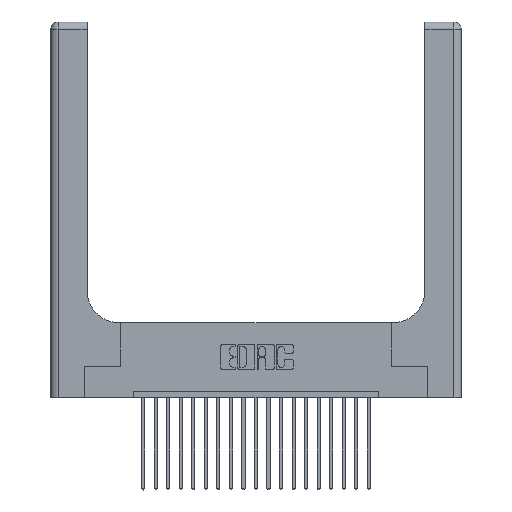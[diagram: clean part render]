
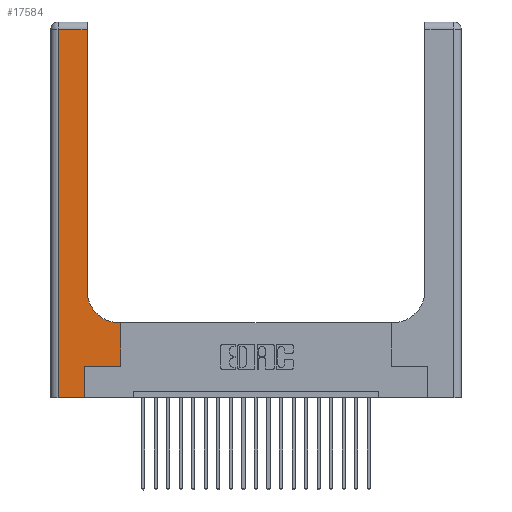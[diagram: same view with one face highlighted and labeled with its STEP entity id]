
A CAD part, top view. The second image highlights one B-rep face of the part: STEP entity #17584.
In plain terms, the highlighted planar face has unit normal (0, 0, 1).
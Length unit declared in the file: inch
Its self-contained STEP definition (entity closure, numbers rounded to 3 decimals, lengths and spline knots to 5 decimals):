
#168 = EDGE_CURVE ( 'NONE', #10191, #3709, #19408, .T. ) ;
#273 = CARTESIAN_POINT ( 'NONE',  ( 0.269, 0.25, 0.37 ) ) ;
#322 = CARTESIAN_POINT ( 'NONE',  ( 0.2915, 3., 0.37 ) ) ;
#757 = DIRECTION ( 'NONE',  ( -1., 0., 0. ) ) ;
#810 = CARTESIAN_POINT ( 'NONE',  ( 0.5585, 0.25, 0.37 ) ) ;
#891 = VERTEX_POINT ( 'NONE', #18353 ) ;
#1217 = VERTEX_POINT ( 'NONE', #17663 ) ;
#1463 = ORIENTED_EDGE ( 'NONE', *, *, #18354, .T. ) ;
#1999 = PLANE ( 'NONE',  #11865 ) ;
#2296 = VERTEX_POINT ( 'NONE', #17834 ) ;
#2933 = CARTESIAN_POINT ( 'NONE',  ( 0.5415, 0.6, 0.37 ) ) ;
#3009 = LINE ( 'NONE', #12864, #11711 ) ;
#3451 = VERTEX_POINT ( 'NONE', #3550 ) ;
#3550 = CARTESIAN_POINT ( 'NONE',  ( 0.5585, 0.25, 0.37 ) ) ;
#3689 = EDGE_CURVE ( 'NONE', #1217, #2296, #17330, .T. ) ;
#3709 = VERTEX_POINT ( 'NONE', #2933 ) ;
#3733 = CARTESIAN_POINT ( 'NONE',  ( 0.5415, 0.85, 0.37 ) ) ;
#3971 = DIRECTION ( 'NONE',  ( 0., 1., 0. ) ) ;
#4291 = DIRECTION ( 'NONE',  ( -1., 0., 0. ) ) ;
#4514 = CARTESIAN_POINT ( 'NONE',  ( 0.269, 0., 0.37 ) ) ;
#4604 = DIRECTION ( 'NONE',  ( 0., -1., 0. ) ) ;
#5093 = EDGE_LOOP ( 'NONE', ( #12547, #1463, #9189, #16789, #19418, #16850, #10582, #7825, #8293 ) ) ;
#5188 = EDGE_CURVE ( 'NONE', #3709, #891, #14259, .T. ) ;
#5521 = DIRECTION ( 'NONE',  ( -1., 0., 0. ) ) ;
#5680 = EDGE_CURVE ( 'NONE', #13908, #3451, #15367, .T. ) ;
#7825 = ORIENTED_EDGE ( 'NONE', *, *, #168, .T. ) ;
#8068 = DIRECTION ( 'NONE',  ( 0., 1., 0. ) ) ;
#8293 = ORIENTED_EDGE ( 'NONE', *, *, #5188, .T. ) ;
#9189 = ORIENTED_EDGE ( 'NONE', *, *, #3689, .T. ) ;
#9375 = EDGE_CURVE ( 'NONE', #891, #15119, #11954, .T. ) ;
#9496 = AXIS2_PLACEMENT_3D ( 'NONE', #3733, #15898, #17657 ) ;
#10011 = DIRECTION ( 'NONE',  ( 1., 0., 0. ) ) ;
#10191 = VERTEX_POINT ( 'NONE', #20766 ) ;
#10582 = ORIENTED_EDGE ( 'NONE', *, *, #22367, .T. ) ;
#10613 = VECTOR ( 'NONE', #10011, 39.37008 ) ;
#11036 = CARTESIAN_POINT ( 'NONE',  ( 0.269, 0., 0.37 ) ) ;
#11158 = LINE ( 'NONE', #20185, #10613 ) ;
#11194 = CARTESIAN_POINT ( 'NONE',  ( 0.269, 0.25, 0.37 ) ) ;
#11668 = VERTEX_POINT ( 'NONE', #4514 ) ;
#11711 = VECTOR ( 'NONE', #757, 39.37008 ) ;
#11865 = AXIS2_PLACEMENT_3D ( 'NONE', #14187, #12590, #5521 ) ;
#11954 = LINE ( 'NONE', #322, #19841 ) ;
#12339 = CARTESIAN_POINT ( 'NONE',  ( 0.2915, 2.94, 0.37 ) ) ;
#12547 = ORIENTED_EDGE ( 'NONE', *, *, #9375, .T. ) ;
#12590 = DIRECTION ( 'NONE',  ( 0., 0., -1. ) ) ;
#12864 = CARTESIAN_POINT ( 'NONE',  ( 0., 2.94, 0.37 ) ) ;
#13506 = CARTESIAN_POINT ( 'NONE',  ( 0.06, 3., 0.37 ) ) ;
#13908 = VERTEX_POINT ( 'NONE', #273 ) ;
#14187 = CARTESIAN_POINT ( 'NONE',  ( 0., 3., 0.37 ) ) ;
#14259 = CIRCLE ( 'NONE', #9496, 0.25 ) ;
#14429 = CARTESIAN_POINT ( 'NONE',  ( 0.2915, 0.6, 0.37 ) ) ;
#14502 = VECTOR ( 'NONE', #4291, 39.37008 ) ;
#15119 = VERTEX_POINT ( 'NONE', #12339 ) ;
#15268 = EDGE_CURVE ( 'NONE', #11668, #13908, #20322, .T. ) ;
#15367 = LINE ( 'NONE', #11194, #19455 ) ;
#15805 = DIRECTION ( 'NONE',  ( 0., 1., 0. ) ) ;
#15898 = DIRECTION ( 'NONE',  ( 0., 0., -1. ) ) ;
#16220 = LINE ( 'NONE', #810, #21674 ) ;
#16789 = ORIENTED_EDGE ( 'NONE', *, *, #18568, .T. ) ;
#16850 = ORIENTED_EDGE ( 'NONE', *, *, #5680, .T. ) ;
#17203 = FACE_OUTER_BOUND ( 'NONE', #5093, .T. ) ;
#17330 = LINE ( 'NONE', #13506, #19518 ) ;
#17584 = ADVANCED_FACE ( 'NONE', ( #17203 ), #1999, .F. ) ;
#17657 = DIRECTION ( 'NONE',  ( 1., 0., 0. ) ) ;
#17663 = CARTESIAN_POINT ( 'NONE',  ( 0.06, 2.94, 0.37 ) ) ;
#17834 = CARTESIAN_POINT ( 'NONE',  ( 0.06, 0., 0.37 ) ) ;
#18353 = CARTESIAN_POINT ( 'NONE',  ( 0.2915, 0.85, 0.37 ) ) ;
#18354 = EDGE_CURVE ( 'NONE', #15119, #1217, #3009, .T. ) ;
#18568 = EDGE_CURVE ( 'NONE', #2296, #11668, #11158, .T. ) ;
#19408 = LINE ( 'NONE', #14429, #14502 ) ;
#19418 = ORIENTED_EDGE ( 'NONE', *, *, #15268, .T. ) ;
#19455 = VECTOR ( 'NONE', #19576, 39.37008 ) ;
#19518 = VECTOR ( 'NONE', #4604, 39.37008 ) ;
#19576 = DIRECTION ( 'NONE',  ( 1., 0., 0. ) ) ;
#19841 = VECTOR ( 'NONE', #15805, 39.37008 ) ;
#20033 = VECTOR ( 'NONE', #3971, 39.37008 ) ;
#20185 = CARTESIAN_POINT ( 'NONE',  ( 0., 0., 0.37 ) ) ;
#20322 = LINE ( 'NONE', #11036, #20033 ) ;
#20766 = CARTESIAN_POINT ( 'NONE',  ( 0.5585, 0.6, 0.37 ) ) ;
#21674 = VECTOR ( 'NONE', #8068, 39.37008 ) ;
#22367 = EDGE_CURVE ( 'NONE', #3451, #10191, #16220, .T. ) ;
